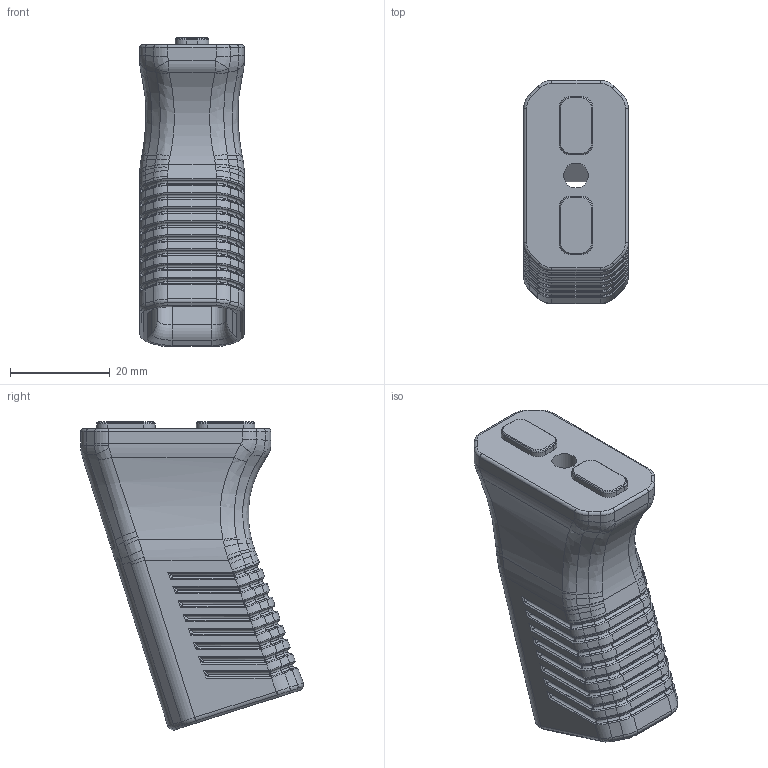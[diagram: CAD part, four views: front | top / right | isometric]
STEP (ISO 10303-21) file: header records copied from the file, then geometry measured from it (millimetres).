
FILE_DESCRIPTION(/* description */ (''),/* implementation_level */ '2;1');
FILE_NAME(/* name */ 'Wrap Ridged.step',/* time_stamp */ '2021-11-24T02:39:45-05:00',/* author */ (''),/* organization */ (''),/* preprocessor_version */ 'ST-DEVELOPER v18.1',/* originating_system */ 'Autodesk Translation Framework v10.10.0.1391',/* authorisation */ '');
FILE_SCHEMA (('AUTOMOTIVE_DESIGN { 1 0 10303 214 3 1 1 }'));
Length unit declared in the file: millimetre
Products named in the file (1): Wrap Ridged
Bounding box: 21 x 44.72 x 61.96 mm (x, y, z)
Volume: 17626.4 mm3; surface area: 10483.5 mm2
Topology: 1 solids, 1 shells, 1113 faces, 2591 edges, 1484 vertices
Faces by surface type: plane 362, cylinder 267, bspline 246, cone 142, torus 94, sphere 2
Full cylindrical faces by diameter (mm): 5 x1
Entity records: 35619 total; most frequent: CARTESIAN_POINT 11445, ORIENTED_EDGE 5174, DIRECTION 4813, EDGE_CURVE 2587, AXIS2_PLACEMENT_3D 1798, VERTEX_POINT 1484, LINE 1217, VECTOR 1217
